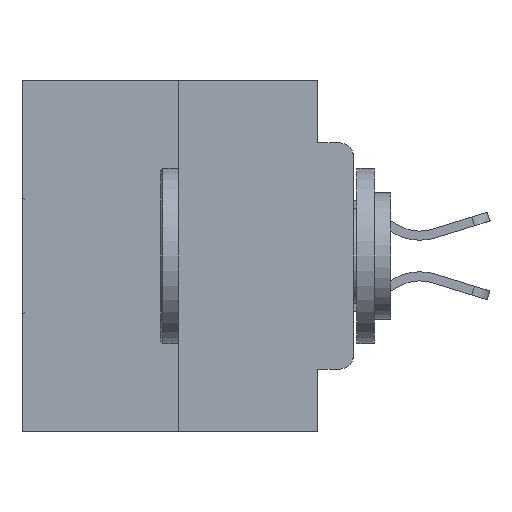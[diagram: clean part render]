
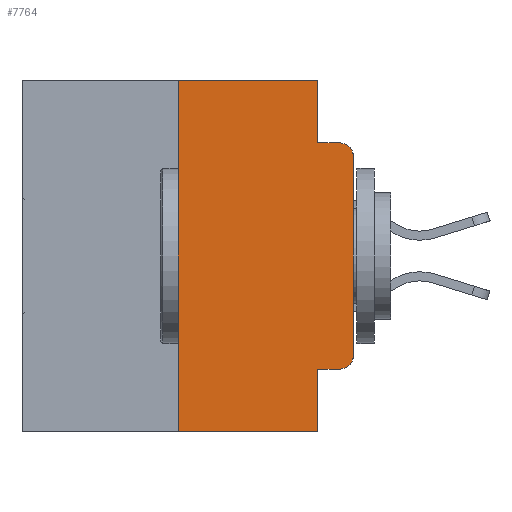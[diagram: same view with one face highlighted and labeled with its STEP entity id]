
A CAD part, left-side view. The second image highlights one B-rep face of the part: STEP entity #7764.
In plain terms, the highlighted planar face has unit normal (-1, 0, 0).
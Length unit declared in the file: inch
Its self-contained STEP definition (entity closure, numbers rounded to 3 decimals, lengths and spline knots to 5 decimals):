
#207 = AXIS2_PLACEMENT_3D ( 'NONE', #21156, #14525, #395 ) ;
#395 = DIRECTION ( 'NONE',  ( 0., 0., -1. ) ) ;
#738 = CARTESIAN_POINT ( 'NONE',  ( 0., 0.051, -0.0885 ) ) ;
#1083 = VERTEX_POINT ( 'NONE', #25291 ) ;
#1552 = CARTESIAN_POINT ( 'NONE',  ( 0., 0.02, -0.1085 ) ) ;
#1816 = DIRECTION ( 'NONE',  ( 0., 0., 1. ) ) ;
#2273 = ORIENTED_EDGE ( 'NONE', *, *, #26197, .F. ) ;
#2619 = CARTESIAN_POINT ( 'NONE',  ( 0., 0.051, -0.4115 ) ) ;
#3071 = EDGE_CURVE ( 'NONE', #25550, #25150, #10129, .T. ) ;
#3122 = CARTESIAN_POINT ( 'NONE',  ( 0., 0.25, -0.5 ) ) ;
#3824 = CARTESIAN_POINT ( 'NONE',  ( 0., 0.051, 0. ) ) ;
#4015 = DIRECTION ( 'NONE',  ( 0., 0., -1. ) ) ;
#4176 = ORIENTED_EDGE ( 'NONE', *, *, #16129, .F. ) ;
#4547 = ORIENTED_EDGE ( 'NONE', *, *, #17239, .T. ) ;
#4707 = EDGE_CURVE ( 'NONE', #22442, #25550, #8982, .T. ) ;
#4829 = VECTOR ( 'NONE', #12021, 39.37008 ) ;
#5206 = PLANE ( 'NONE',  #207 ) ;
#5211 = DIRECTION ( 'NONE',  ( -1., 0., 0. ) ) ;
#5273 = ORIENTED_EDGE ( 'NONE', *, *, #3071, .T. ) ;
#5428 = VECTOR ( 'NONE', #25652, 39.37008 ) ;
#5819 = LINE ( 'NONE', #11211, #11987 ) ;
#6494 = LINE ( 'NONE', #19069, #11931 ) ;
#7157 = VERTEX_POINT ( 'NONE', #21085 ) ;
#7351 = CARTESIAN_POINT ( 'NONE',  ( 0., 0.473, -0.5 ) ) ;
#7479 = CARTESIAN_POINT ( 'NONE',  ( 0., 0.051, -0.4115 ) ) ;
#7764 = ADVANCED_FACE ( 'NONE', ( #28172 ), #5206, .F. ) ;
#8115 = VECTOR ( 'NONE', #12524, 39.37008 ) ;
#8555 = ORIENTED_EDGE ( 'NONE', *, *, #4707, .T. ) ;
#8744 = LINE ( 'NONE', #3824, #19416 ) ;
#8850 = LINE ( 'NONE', #738, #8115 ) ;
#8982 = LINE ( 'NONE', #23284, #10446 ) ;
#8995 = CARTESIAN_POINT ( 'NONE',  ( 0., 0.051, -0.0885 ) ) ;
#9087 = CARTESIAN_POINT ( 'NONE',  ( 0., 0., -0.3915 ) ) ;
#10129 = CIRCLE ( 'NONE', #17921, 0.02 ) ;
#10387 = ORIENTED_EDGE ( 'NONE', *, *, #27136, .F. ) ;
#10446 = VECTOR ( 'NONE', #18811, 39.37008 ) ;
#10985 = DIRECTION ( 'NONE',  ( 0., 0., -1. ) ) ;
#11039 = LINE ( 'NONE', #7351, #4829 ) ;
#11211 = CARTESIAN_POINT ( 'NONE',  ( 0., 0.25, 0. ) ) ;
#11931 = VECTOR ( 'NONE', #23443, 39.37008 ) ;
#11987 = VECTOR ( 'NONE', #1816, 39.37008 ) ;
#12021 = DIRECTION ( 'NONE',  ( 0., -1., 0. ) ) ;
#12524 = DIRECTION ( 'NONE',  ( 0., -1., 0. ) ) ;
#13990 = CIRCLE ( 'NONE', #26634, 0.02 ) ;
#14403 = VERTEX_POINT ( 'NONE', #2619 ) ;
#14525 = DIRECTION ( 'NONE',  ( 1., 0., 0. ) ) ;
#14537 = CARTESIAN_POINT ( 'NONE',  ( 0., 0.473, 0. ) ) ;
#15527 = CARTESIAN_POINT ( 'NONE',  ( 0., 0., -0.1085 ) ) ;
#15810 = VERTEX_POINT ( 'NONE', #8995 ) ;
#15994 = EDGE_CURVE ( 'NONE', #17445, #27562, #11039, .T. ) ;
#16129 = EDGE_CURVE ( 'NONE', #15810, #25150, #8850, .T. ) ;
#16843 = ORIENTED_EDGE ( 'NONE', *, *, #26445, .T. ) ;
#17239 = EDGE_CURVE ( 'NONE', #14403, #7157, #19102, .T. ) ;
#17445 = VERTEX_POINT ( 'NONE', #3122 ) ;
#17810 = DIRECTION ( 'NONE',  ( -1., 0., 0. ) ) ;
#17921 = AXIS2_PLACEMENT_3D ( 'NONE', #1552, #17810, #4015 ) ;
#18174 = EDGE_CURVE ( 'NONE', #1083, #19739, #22862, .T. ) ;
#18375 = CARTESIAN_POINT ( 'NONE',  ( 0., 0.02, -0.0885 ) ) ;
#18465 = CARTESIAN_POINT ( 'NONE',  ( 0., 0.051, -0.5 ) ) ;
#18811 = DIRECTION ( 'NONE',  ( 0., 0., 1. ) ) ;
#18928 = CARTESIAN_POINT ( 'NONE',  ( 0., 0.02, -0.3915 ) ) ;
#19069 = CARTESIAN_POINT ( 'NONE',  ( 0., 0.051, 0. ) ) ;
#19102 = LINE ( 'NONE', #7479, #24330 ) ;
#19416 = VECTOR ( 'NONE', #10985, 39.37008 ) ;
#19739 = VERTEX_POINT ( 'NONE', #22248 ) ;
#19957 = ORIENTED_EDGE ( 'NONE', *, *, #15994, .T. ) ;
#21085 = CARTESIAN_POINT ( 'NONE',  ( 0., 0.02, -0.4115 ) ) ;
#21156 = CARTESIAN_POINT ( 'NONE',  ( 0., 0.473, 0. ) ) ;
#21158 = DIRECTION ( 'NONE',  ( 0., 0., -1. ) ) ;
#21632 = EDGE_LOOP ( 'NONE', ( #8555, #5273, #4176, #10387, #23078, #28995, #19957, #2273, #4547, #16843 ) ) ;
#22248 = CARTESIAN_POINT ( 'NONE',  ( 0., 0.051, 0. ) ) ;
#22442 = VERTEX_POINT ( 'NONE', #9087 ) ;
#22862 = LINE ( 'NONE', #14537, #5428 ) ;
#23078 = ORIENTED_EDGE ( 'NONE', *, *, #18174, .F. ) ;
#23284 = CARTESIAN_POINT ( 'NONE',  ( 0., 0., 0. ) ) ;
#23344 = DIRECTION ( 'NONE',  ( 0., -1., 0. ) ) ;
#23443 = DIRECTION ( 'NONE',  ( 0., 0., -1. ) ) ;
#24330 = VECTOR ( 'NONE', #23344, 39.37008 ) ;
#25150 = VERTEX_POINT ( 'NONE', #18375 ) ;
#25291 = CARTESIAN_POINT ( 'NONE',  ( 0., 0.25, 0. ) ) ;
#25550 = VERTEX_POINT ( 'NONE', #15527 ) ;
#25630 = EDGE_CURVE ( 'NONE', #17445, #1083, #5819, .T. ) ;
#25652 = DIRECTION ( 'NONE',  ( 0., -1., 0. ) ) ;
#26197 = EDGE_CURVE ( 'NONE', #14403, #27562, #8744, .T. ) ;
#26445 = EDGE_CURVE ( 'NONE', #7157, #22442, #13990, .T. ) ;
#26634 = AXIS2_PLACEMENT_3D ( 'NONE', #18928, #5211, #21158 ) ;
#27136 = EDGE_CURVE ( 'NONE', #19739, #15810, #6494, .T. ) ;
#27562 = VERTEX_POINT ( 'NONE', #18465 ) ;
#28172 = FACE_OUTER_BOUND ( 'NONE', #21632, .T. ) ;
#28995 = ORIENTED_EDGE ( 'NONE', *, *, #25630, .F. ) ;
